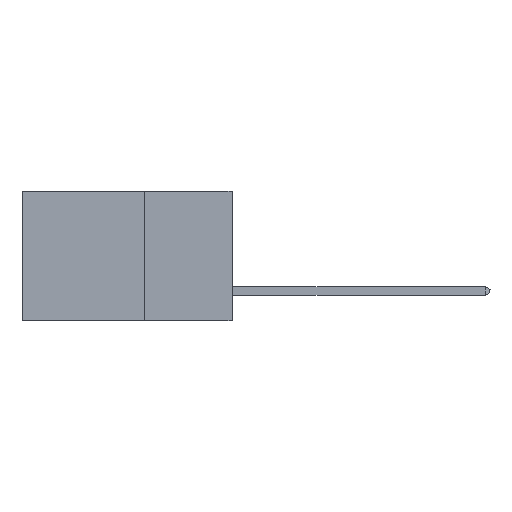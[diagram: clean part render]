
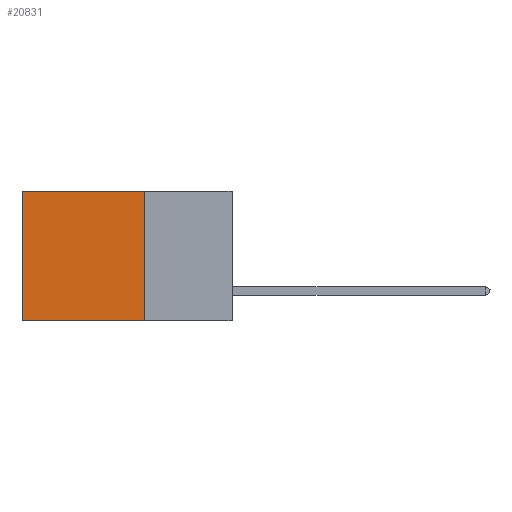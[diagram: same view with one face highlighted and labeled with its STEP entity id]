
A CAD part, left-side view. The second image highlights one B-rep face of the part: STEP entity #20831.
In plain terms, the highlighted planar face has unit normal (-1, 0, 0).
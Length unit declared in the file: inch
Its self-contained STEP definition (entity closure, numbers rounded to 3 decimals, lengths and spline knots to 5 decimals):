
#966 = DIRECTION ( 'NONE',  ( 0., 0., -1. ) ) ;
#1573 = LINE ( 'NONE', #4981, #21816 ) ;
#1793 = CARTESIAN_POINT ( 'NONE',  ( 0.2875, 0.6, 0. ) ) ;
#2128 = DIRECTION ( 'NONE',  ( 0., 1., 0. ) ) ;
#2279 = VECTOR ( 'NONE', #2128, 39.37008 ) ;
#2675 = EDGE_CURVE ( 'NONE', #18135, #14845, #18516, .T. ) ;
#3492 = ORIENTED_EDGE ( 'NONE', *, *, #9869, .F. ) ;
#3507 = DIRECTION ( 'NONE',  ( 0., 0., -1. ) ) ;
#4719 = LINE ( 'NONE', #17774, #14191 ) ;
#4981 = CARTESIAN_POINT ( 'NONE',  ( 0.2875, 0.25, 0. ) ) ;
#6418 = CARTESIAN_POINT ( 'NONE',  ( 0.2875, 0.25, 0. ) ) ;
#7489 = ORIENTED_EDGE ( 'NONE', *, *, #17467, .F. ) ;
#8202 = PLANE ( 'NONE',  #22534 ) ;
#9723 = CARTESIAN_POINT ( 'NONE',  ( 0.2875, 0.25, -0.37 ) ) ;
#9869 = EDGE_CURVE ( 'NONE', #18135, #19614, #1573, .T. ) ;
#10267 = VECTOR ( 'NONE', #23600, 39.37008 ) ;
#10344 = CARTESIAN_POINT ( 'NONE',  ( 0.2875, 0.25, 0. ) ) ;
#11193 = EDGE_CURVE ( 'NONE', #14845, #21435, #20097, .T. ) ;
#11948 = EDGE_LOOP ( 'NONE', ( #16584, #7489, #3492, #12949 ) ) ;
#12949 = ORIENTED_EDGE ( 'NONE', *, *, #2675, .T. ) ;
#13020 = CARTESIAN_POINT ( 'NONE',  ( 0.2875, 0.25, 0. ) ) ;
#14027 = CARTESIAN_POINT ( 'NONE',  ( 0.2875, 0.6, 0. ) ) ;
#14191 = VECTOR ( 'NONE', #19524, 39.37008 ) ;
#14845 = VERTEX_POINT ( 'NONE', #14027 ) ;
#16584 = ORIENTED_EDGE ( 'NONE', *, *, #11193, .T. ) ;
#17467 = EDGE_CURVE ( 'NONE', #19614, #21435, #4719, .T. ) ;
#17774 = CARTESIAN_POINT ( 'NONE',  ( 0.2875, 0.25, -0.37 ) ) ;
#18135 = VERTEX_POINT ( 'NONE', #6418 ) ;
#18516 = LINE ( 'NONE', #13020, #2279 ) ;
#19029 = CARTESIAN_POINT ( 'NONE',  ( 0.2875, 0.6, -0.37 ) ) ;
#19524 = DIRECTION ( 'NONE',  ( 0., 1., 0. ) ) ;
#19537 = DIRECTION ( 'NONE',  ( 1., 0., 0. ) ) ;
#19614 = VERTEX_POINT ( 'NONE', #9723 ) ;
#20097 = LINE ( 'NONE', #1793, #10267 ) ;
#20831 = ADVANCED_FACE ( 'NONE', ( #21791 ), #8202, .F. ) ;
#21435 = VERTEX_POINT ( 'NONE', #19029 ) ;
#21791 = FACE_OUTER_BOUND ( 'NONE', #11948, .T. ) ;
#21816 = VECTOR ( 'NONE', #3507, 39.37008 ) ;
#22534 = AXIS2_PLACEMENT_3D ( 'NONE', #10344, #19537, #966 ) ;
#23600 = DIRECTION ( 'NONE',  ( 0., 0., -1. ) ) ;
